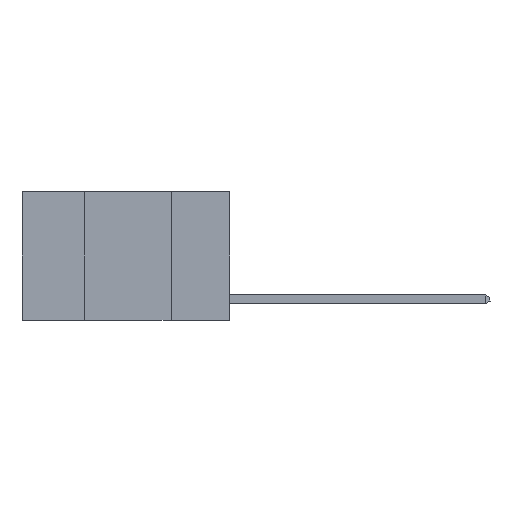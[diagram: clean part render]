
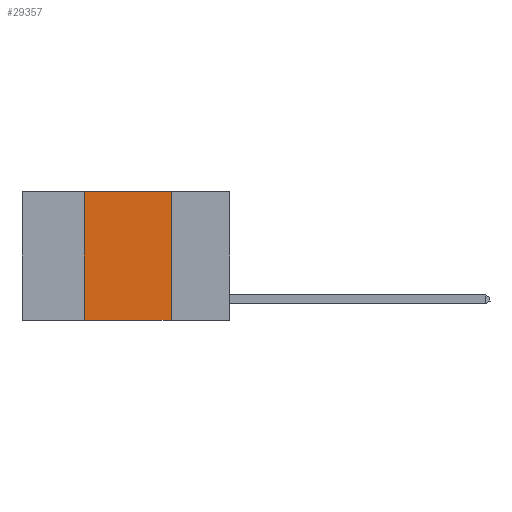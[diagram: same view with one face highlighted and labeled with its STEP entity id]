
A CAD part, left-side view. The second image highlights one B-rep face of the part: STEP entity #29357.
In plain terms, the highlighted planar face has unit normal (-1, 0, 0).
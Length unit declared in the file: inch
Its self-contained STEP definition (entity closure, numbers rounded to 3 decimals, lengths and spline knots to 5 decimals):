
#1212 = LINE ( 'NONE', #13323, #15867 ) ;
#1536 = LINE ( 'NONE', #6546, #26583 ) ;
#2006 = VERTEX_POINT ( 'NONE', #26945 ) ;
#3248 = VECTOR ( 'NONE', #29384, 39.37008 ) ;
#5170 = VERTEX_POINT ( 'NONE', #27653 ) ;
#5286 = EDGE_CURVE ( 'NONE', #16462, #9551, #11051, .T. ) ;
#5605 = PLANE ( 'NONE',  #13982 ) ;
#5645 = CARTESIAN_POINT ( 'NONE',  ( 0., 0.17, 0. ) ) ;
#6308 = EDGE_CURVE ( 'NONE', #2006, #5170, #8988, .T. ) ;
#6546 = CARTESIAN_POINT ( 'NONE',  ( 0., 0.6, 0. ) ) ;
#7692 = DIRECTION ( 'NONE',  ( 1., 0., 0. ) ) ;
#8267 = CARTESIAN_POINT ( 'NONE',  ( 0., 0.42, 0. ) ) ;
#8988 = LINE ( 'NONE', #8267, #3248 ) ;
#9551 = VERTEX_POINT ( 'NONE', #23032 ) ;
#10558 = EDGE_CURVE ( 'NONE', #5170, #16462, #1536, .T. ) ;
#10800 = ORIENTED_EDGE ( 'NONE', *, *, #21286, .T. ) ;
#10883 = DIRECTION ( 'NONE',  ( 0., 0., -1. ) ) ;
#11051 = LINE ( 'NONE', #19988, #16448 ) ;
#12507 = CARTESIAN_POINT ( 'NONE',  ( 0., 0.6, 0. ) ) ;
#13173 = EDGE_LOOP ( 'NONE', ( #22649, #13696, #18322, #10800 ) ) ;
#13323 = CARTESIAN_POINT ( 'NONE',  ( 0., 0.6, -0.37 ) ) ;
#13696 = ORIENTED_EDGE ( 'NONE', *, *, #10558, .F. ) ;
#13982 = AXIS2_PLACEMENT_3D ( 'NONE', #12507, #7692, #28463 ) ;
#15806 = FACE_OUTER_BOUND ( 'NONE', #13173, .T. ) ;
#15831 = DIRECTION ( 'NONE',  ( 0., -1., 0. ) ) ;
#15867 = VECTOR ( 'NONE', #15831, 39.37008 ) ;
#16448 = VECTOR ( 'NONE', #10883, 39.37008 ) ;
#16462 = VERTEX_POINT ( 'NONE', #5645 ) ;
#18322 = ORIENTED_EDGE ( 'NONE', *, *, #6308, .F. ) ;
#19988 = CARTESIAN_POINT ( 'NONE',  ( 0., 0.17, 0. ) ) ;
#20129 = DIRECTION ( 'NONE',  ( 0., -1., 0. ) ) ;
#21286 = EDGE_CURVE ( 'NONE', #2006, #9551, #1212, .T. ) ;
#22649 = ORIENTED_EDGE ( 'NONE', *, *, #5286, .F. ) ;
#23032 = CARTESIAN_POINT ( 'NONE',  ( 0., 0.17, -0.37 ) ) ;
#26583 = VECTOR ( 'NONE', #20129, 39.37008 ) ;
#26945 = CARTESIAN_POINT ( 'NONE',  ( 0., 0.42, -0.37 ) ) ;
#27653 = CARTESIAN_POINT ( 'NONE',  ( 0., 0.42, 0. ) ) ;
#28463 = DIRECTION ( 'NONE',  ( 0., 0., -1. ) ) ;
#29357 = ADVANCED_FACE ( 'NONE', ( #15806 ), #5605, .F. ) ;
#29384 = DIRECTION ( 'NONE',  ( 0., 0., 1. ) ) ;
